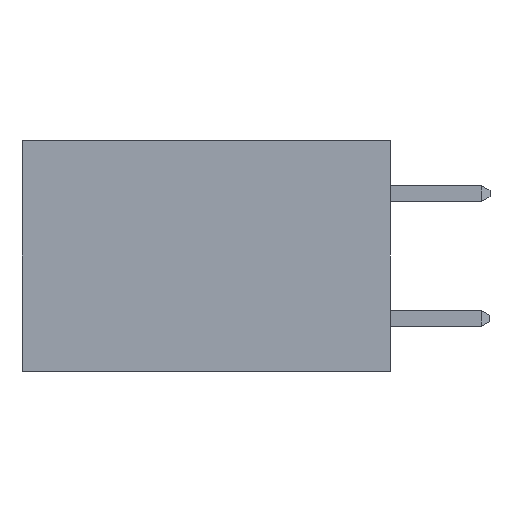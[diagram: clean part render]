
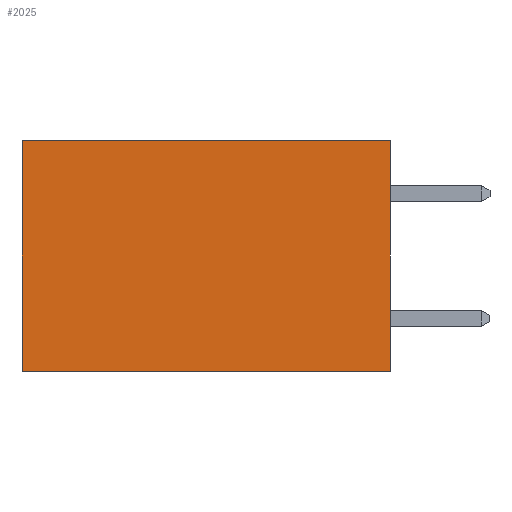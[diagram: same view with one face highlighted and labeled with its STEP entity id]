
A CAD part, left-side view. The second image highlights one B-rep face of the part: STEP entity #2025.
In plain terms, the highlighted planar face has unit normal (-1, 0, 0).
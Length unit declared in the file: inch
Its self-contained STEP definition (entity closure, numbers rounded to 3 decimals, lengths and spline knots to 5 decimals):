
#425 = CARTESIAN_POINT ( 'NONE',  ( 0.277, 0.59, 0. ) ) ;
#449 = VERTEX_POINT ( 'NONE', #4346 ) ;
#507 = LINE ( 'NONE', #5312, #7591 ) ;
#589 = CARTESIAN_POINT ( 'NONE',  ( 0.277, 0., -0.37 ) ) ;
#668 = DIRECTION ( 'NONE',  ( 0., 0., -1. ) ) ;
#674 = DIRECTION ( 'NONE',  ( 1., 0., 0. ) ) ;
#804 = PLANE ( 'NONE',  #6300 ) ;
#1153 = CARTESIAN_POINT ( 'NONE',  ( 0.277, 0., -0.37 ) ) ;
#1740 = FACE_OUTER_BOUND ( 'NONE', #4077, .T. ) ;
#2025 = ADVANCED_FACE ( 'NONE', ( #1740 ), #804, .F. ) ;
#2443 = DIRECTION ( 'NONE',  ( 0., 0., -1. ) ) ;
#2675 = ORIENTED_EDGE ( 'NONE', *, *, #6992, .T. ) ;
#2796 = VECTOR ( 'NONE', #3376, 39.37008 ) ;
#2824 = VERTEX_POINT ( 'NONE', #425 ) ;
#2848 = CARTESIAN_POINT ( 'NONE',  ( 0.277, 0., -0.37 ) ) ;
#2952 = ORIENTED_EDGE ( 'NONE', *, *, #7511, .F. ) ;
#3212 = CARTESIAN_POINT ( 'NONE',  ( 0.277, 0.59, -0.37 ) ) ;
#3376 = DIRECTION ( 'NONE',  ( 0., 0., -1. ) ) ;
#3455 = ORIENTED_EDGE ( 'NONE', *, *, #5236, .F. ) ;
#3826 = ORIENTED_EDGE ( 'NONE', *, *, #6389, .T. ) ;
#3853 = CARTESIAN_POINT ( 'NONE',  ( 0.277, 0., -0.37 ) ) ;
#4077 = EDGE_LOOP ( 'NONE', ( #2675, #2952, #3455, #3826 ) ) ;
#4346 = CARTESIAN_POINT ( 'NONE',  ( 0.277, 0., 0. ) ) ;
#4511 = CARTESIAN_POINT ( 'NONE',  ( 0.277, 0., 0. ) ) ;
#4793 = DIRECTION ( 'NONE',  ( 0., 1., 0. ) ) ;
#5173 = VERTEX_POINT ( 'NONE', #3212 ) ;
#5236 = EDGE_CURVE ( 'NONE', #449, #5766, #5839, .T. ) ;
#5312 = CARTESIAN_POINT ( 'NONE',  ( 0.277, 0.59, -0.37 ) ) ;
#5461 = LINE ( 'NONE', #2848, #6825 ) ;
#5480 = LINE ( 'NONE', #4511, #6843 ) ;
#5766 = VERTEX_POINT ( 'NONE', #589 ) ;
#5839 = LINE ( 'NONE', #3853, #2796 ) ;
#6284 = DIRECTION ( 'NONE',  ( 0., 1., 0. ) ) ;
#6300 = AXIS2_PLACEMENT_3D ( 'NONE', #1153, #674, #668 ) ;
#6389 = EDGE_CURVE ( 'NONE', #449, #2824, #5480, .T. ) ;
#6825 = VECTOR ( 'NONE', #6284, 39.37008 ) ;
#6843 = VECTOR ( 'NONE', #4793, 39.37008 ) ;
#6992 = EDGE_CURVE ( 'NONE', #2824, #5173, #507, .T. ) ;
#7511 = EDGE_CURVE ( 'NONE', #5766, #5173, #5461, .T. ) ;
#7591 = VECTOR ( 'NONE', #2443, 39.37008 ) ;
